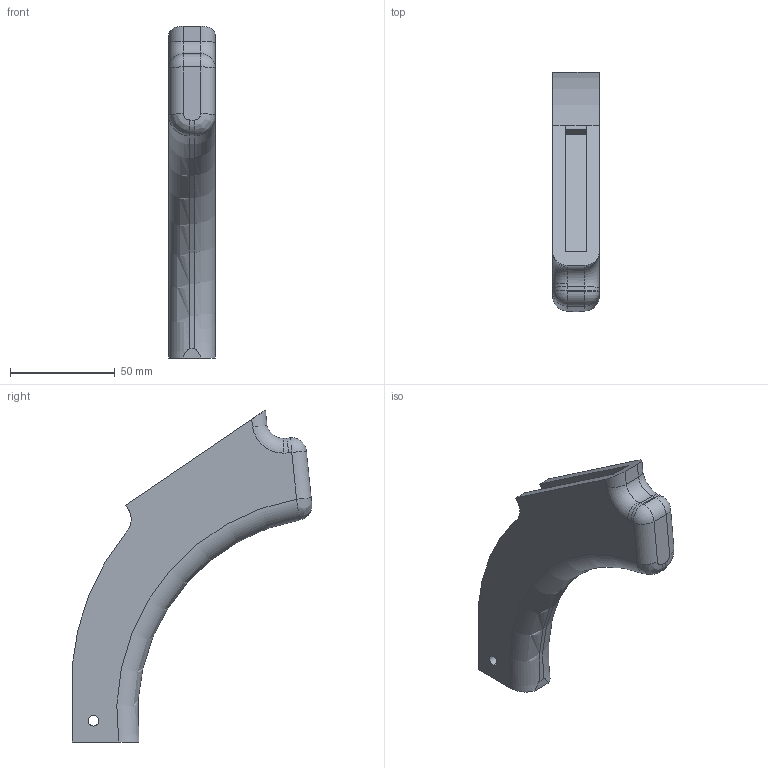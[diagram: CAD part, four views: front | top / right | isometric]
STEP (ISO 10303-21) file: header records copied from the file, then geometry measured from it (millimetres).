
FILE_DESCRIPTION (( 'STEP AP214' ), '1' );
FILE_NAME ('hydrastockx1.STEP', '2013-07-04T02:27:05', ( '' ), ( '' ), 'SwSTEP 2.0', 'SolidWorks 2012', '' );
FILE_SCHEMA (( 'AUTOMOTIVE_DESIGN' ));
Length unit declared in the file: millimetre
Products named in the file (1): hydrastockx1
Bounding box: 22.24 x 114.4 x 158.48 mm (x, y, z)
Volume: 139504.1 mm3; surface area: 24866.7 mm2
Topology: 1 solids, 1 shells, 51 faces, 130 edges, 81 vertices
Faces by surface type: plane 24, cylinder 17, torus 5, sphere 3, bspline 2
Entity records: 1926 total; most frequent: CARTESIAN_POINT 660, ORIENTED_EDGE 260, DIRECTION 254, EDGE_CURVE 130, AXIS2_PLACEMENT_3D 89, VERTEX_POINT 81, LINE 76, VECTOR 76
